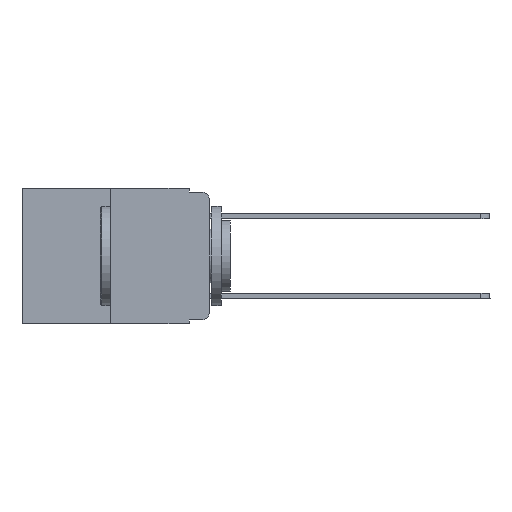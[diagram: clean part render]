
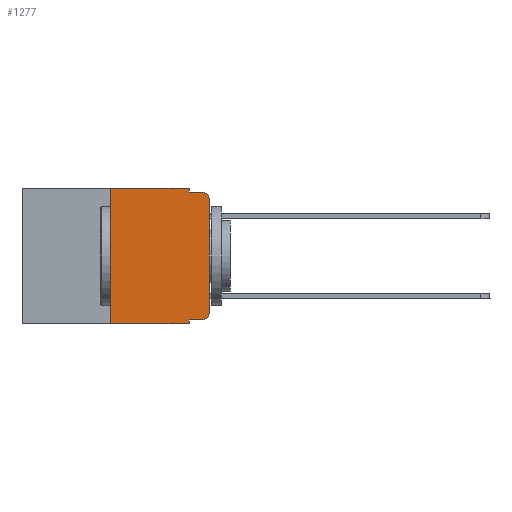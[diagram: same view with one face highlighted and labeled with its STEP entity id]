
A CAD part, left-side view. The second image highlights one B-rep face of the part: STEP entity #1277.
In plain terms, the highlighted planar face has unit normal (-1, 0, 0).
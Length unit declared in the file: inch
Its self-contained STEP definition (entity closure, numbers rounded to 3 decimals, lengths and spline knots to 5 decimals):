
#20 = EDGE_CURVE ( 'NONE', #1043, #868, #5177, .T. ) ;
#66 = LINE ( 'NONE', #10017, #7434 ) ;
#133 = EDGE_CURVE ( 'NONE', #10194, #10783, #10717, .T. ) ;
#357 = ORIENTED_EDGE ( 'NONE', *, *, #7512, .F. ) ;
#502 = CARTESIAN_POINT ( 'NONE',  ( 0., 0.473, 0. ) ) ;
#635 = CARTESIAN_POINT ( 'NONE',  ( 0., 0.051, -0.01 ) ) ;
#728 = ORIENTED_EDGE ( 'NONE', *, *, #10981, .T. ) ;
#741 = DIRECTION ( 'NONE',  ( 0., -1., 0. ) ) ;
#765 = AXIS2_PLACEMENT_3D ( 'NONE', #6260, #14677, #7471 ) ;
#776 = CIRCLE ( 'NONE', #15055, 0.02 ) ;
#868 = VERTEX_POINT ( 'NONE', #6745 ) ;
#981 = DIRECTION ( 'NONE',  ( 0., 0., -1. ) ) ;
#1043 = VERTEX_POINT ( 'NONE', #14209 ) ;
#1277 = ADVANCED_FACE ( 'NONE', ( #14047 ), #2740, .F. ) ;
#2220 = CARTESIAN_POINT ( 'NONE',  ( 0., 0.02, -0.01 ) ) ;
#2422 = ORIENTED_EDGE ( 'NONE', *, *, #3212, .T. ) ;
#2485 = ORIENTED_EDGE ( 'NONE', *, *, #12854, .F. ) ;
#2740 = PLANE ( 'NONE',  #765 ) ;
#2757 = VERTEX_POINT ( 'NONE', #12995 ) ;
#2990 = CARTESIAN_POINT ( 'NONE',  ( 0., 0., -0.03 ) ) ;
#3096 = DIRECTION ( 'NONE',  ( 0., 0., -1. ) ) ;
#3125 = VECTOR ( 'NONE', #14720, 39.37008 ) ;
#3212 = EDGE_CURVE ( 'NONE', #14560, #10194, #6889, .T. ) ;
#3290 = ORIENTED_EDGE ( 'NONE', *, *, #8429, .T. ) ;
#3475 = AXIS2_PLACEMENT_3D ( 'NONE', #15346, #6823, #981 ) ;
#3622 = CARTESIAN_POINT ( 'NONE',  ( 0., 0.473, -0.343 ) ) ;
#3697 = VECTOR ( 'NONE', #12796, 39.37008 ) ;
#3955 = CARTESIAN_POINT ( 'NONE',  ( 0., 0.051, -0.343 ) ) ;
#4155 = CARTESIAN_POINT ( 'NONE',  ( 0., 0.25, 0. ) ) ;
#5133 = LINE ( 'NONE', #4155, #7321 ) ;
#5177 = LINE ( 'NONE', #502, #3125 ) ;
#5214 = EDGE_CURVE ( 'NONE', #868, #13895, #66, .T. ) ;
#5390 = CARTESIAN_POINT ( 'NONE',  ( 0., 0.02, -0.333 ) ) ;
#5397 = DIRECTION ( 'NONE',  ( 0., 0., 1. ) ) ;
#5580 = CARTESIAN_POINT ( 'NONE',  ( 0., 0., 0. ) ) ;
#6260 = CARTESIAN_POINT ( 'NONE',  ( 0., 0.473, 0. ) ) ;
#6443 = CARTESIAN_POINT ( 'NONE',  ( 0., 0., -0.313 ) ) ;
#6557 = VECTOR ( 'NONE', #741, 39.37008 ) ;
#6606 = DIRECTION ( 'NONE',  ( 0., 0., -1. ) ) ;
#6745 = CARTESIAN_POINT ( 'NONE',  ( 0., 0.051, 0. ) ) ;
#6779 = DIRECTION ( 'NONE',  ( -1., 0., 0. ) ) ;
#6823 = DIRECTION ( 'NONE',  ( -1., 0., 0. ) ) ;
#6837 = LINE ( 'NONE', #8056, #3697 ) ;
#6889 = CIRCLE ( 'NONE', #3475, 0.02 ) ;
#7321 = VECTOR ( 'NONE', #5397, 39.37008 ) ;
#7332 = VERTEX_POINT ( 'NONE', #13829 ) ;
#7355 = EDGE_CURVE ( 'NONE', #10783, #14843, #776, .T. ) ;
#7434 = VECTOR ( 'NONE', #6606, 39.37008 ) ;
#7471 = DIRECTION ( 'NONE',  ( 0., 0., -1. ) ) ;
#7480 = VECTOR ( 'NONE', #11832, 39.37008 ) ;
#7512 = EDGE_CURVE ( 'NONE', #7332, #7660, #12281, .T. ) ;
#7660 = VERTEX_POINT ( 'NONE', #3955 ) ;
#7916 = DIRECTION ( 'NONE',  ( 0., 0., 1. ) ) ;
#8056 = CARTESIAN_POINT ( 'NONE',  ( 0., 0.051, -0.333 ) ) ;
#8429 = EDGE_CURVE ( 'NONE', #7332, #14560, #6837, .T. ) ;
#8935 = ORIENTED_EDGE ( 'NONE', *, *, #133, .T. ) ;
#9032 = CARTESIAN_POINT ( 'NONE',  ( 0., 0.02, -0.03 ) ) ;
#10017 = CARTESIAN_POINT ( 'NONE',  ( 0., 0.051, 0. ) ) ;
#10022 = VECTOR ( 'NONE', #13991, 39.37008 ) ;
#10194 = VERTEX_POINT ( 'NONE', #6443 ) ;
#10301 = EDGE_CURVE ( 'NONE', #2757, #1043, #5133, .T. ) ;
#10717 = LINE ( 'NONE', #5580, #14317 ) ;
#10783 = VERTEX_POINT ( 'NONE', #2990 ) ;
#10981 = EDGE_CURVE ( 'NONE', #2757, #7660, #15008, .T. ) ;
#11348 = ORIENTED_EDGE ( 'NONE', *, *, #5214, .F. ) ;
#11832 = DIRECTION ( 'NONE',  ( 0., -1., 0. ) ) ;
#12281 = LINE ( 'NONE', #13029, #10022 ) ;
#12343 = LINE ( 'NONE', #635, #6557 ) ;
#12545 = EDGE_LOOP ( 'NONE', ( #8935, #14850, #2485, #11348, #13191, #12856, #728, #357, #3290, #2422 ) ) ;
#12796 = DIRECTION ( 'NONE',  ( 0., -1., 0. ) ) ;
#12854 = EDGE_CURVE ( 'NONE', #13895, #14843, #12343, .T. ) ;
#12856 = ORIENTED_EDGE ( 'NONE', *, *, #10301, .F. ) ;
#12995 = CARTESIAN_POINT ( 'NONE',  ( 0., 0.25, -0.343 ) ) ;
#13029 = CARTESIAN_POINT ( 'NONE',  ( 0., 0.051, 0. ) ) ;
#13191 = ORIENTED_EDGE ( 'NONE', *, *, #20, .F. ) ;
#13597 = CARTESIAN_POINT ( 'NONE',  ( 0., 0.051, -0.01 ) ) ;
#13829 = CARTESIAN_POINT ( 'NONE',  ( 0., 0.051, -0.333 ) ) ;
#13895 = VERTEX_POINT ( 'NONE', #13597 ) ;
#13991 = DIRECTION ( 'NONE',  ( 0., 0., -1. ) ) ;
#14047 = FACE_OUTER_BOUND ( 'NONE', #12545, .T. ) ;
#14209 = CARTESIAN_POINT ( 'NONE',  ( 0., 0.25, 0. ) ) ;
#14317 = VECTOR ( 'NONE', #7916, 39.37008 ) ;
#14560 = VERTEX_POINT ( 'NONE', #5390 ) ;
#14677 = DIRECTION ( 'NONE',  ( 1., 0., 0. ) ) ;
#14720 = DIRECTION ( 'NONE',  ( 0., -1., 0. ) ) ;
#14843 = VERTEX_POINT ( 'NONE', #2220 ) ;
#14850 = ORIENTED_EDGE ( 'NONE', *, *, #7355, .T. ) ;
#15008 = LINE ( 'NONE', #3622, #7480 ) ;
#15055 = AXIS2_PLACEMENT_3D ( 'NONE', #9032, #6779, #3096 ) ;
#15346 = CARTESIAN_POINT ( 'NONE',  ( 0., 0.02, -0.313 ) ) ;
